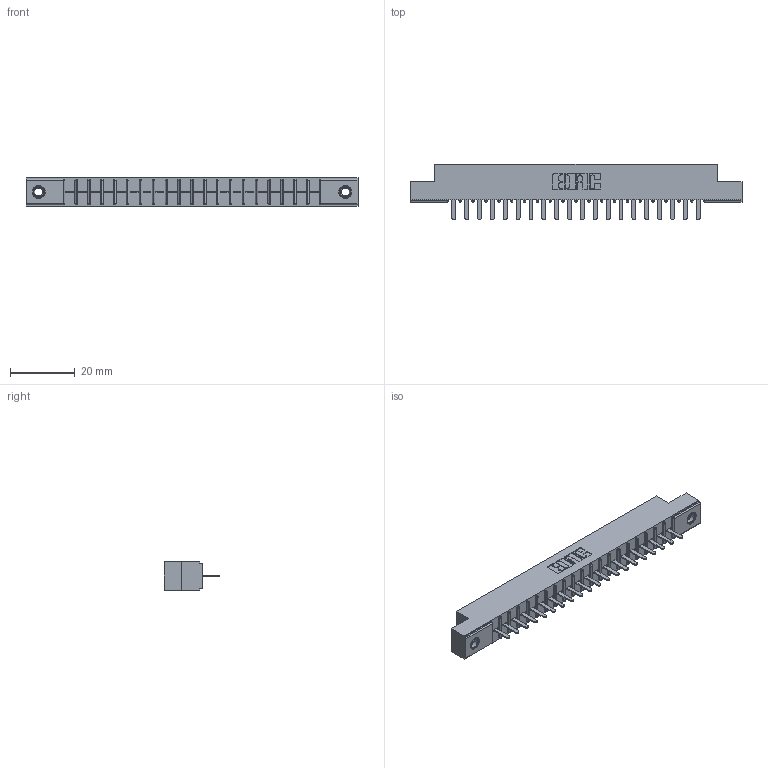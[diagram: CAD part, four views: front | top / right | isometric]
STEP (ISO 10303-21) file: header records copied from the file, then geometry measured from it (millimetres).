
FILE_DESCRIPTION (( 'STEP AP203' ), '1' );
FILE_NAME ('356-020-420-107.STEP', '2020-09-23T14:27:25', ( '' ), ( '' ), 'SwSTEP 2.0', 'SolidWorks 2020', '' );
FILE_SCHEMA (( 'CONFIG_CONTROL_DESIGN' ));
Length unit declared in the file: inch
Products named in the file (4): 306-290-001_120; 345-250-001_345-250-005-103; 356-020-420-107; 306 Part_.156 Dia
Assembly tree (23 placements, depth 2):
  356-020-420-107
    306 Part_.156 Dia
    306-290-001_120  x20
    345-250-001_345-250-005-103  x2
Bounding box: 102.26 x 17.12 x 8.71 mm (x, y, z)
Volume: 6970.4 mm3; surface area: 10293.5 mm2
Topology: 23 solids, 23 shells, 1576 faces, 4392 edges, 2812 vertices
Faces by surface type: plane 1040, cylinder 440, sphere 80, cone 12, torus 4
Entity records: 22642 total; most frequent: CARTESIAN_POINT 3778, ORIENTED_EDGE 3736, DIRECTION 3736, EDGE_CURVE 1868, LINE 1448, VECTOR 1448, VERTEX_POINT 1186, AXIS2_PLACEMENT_3D 1144
